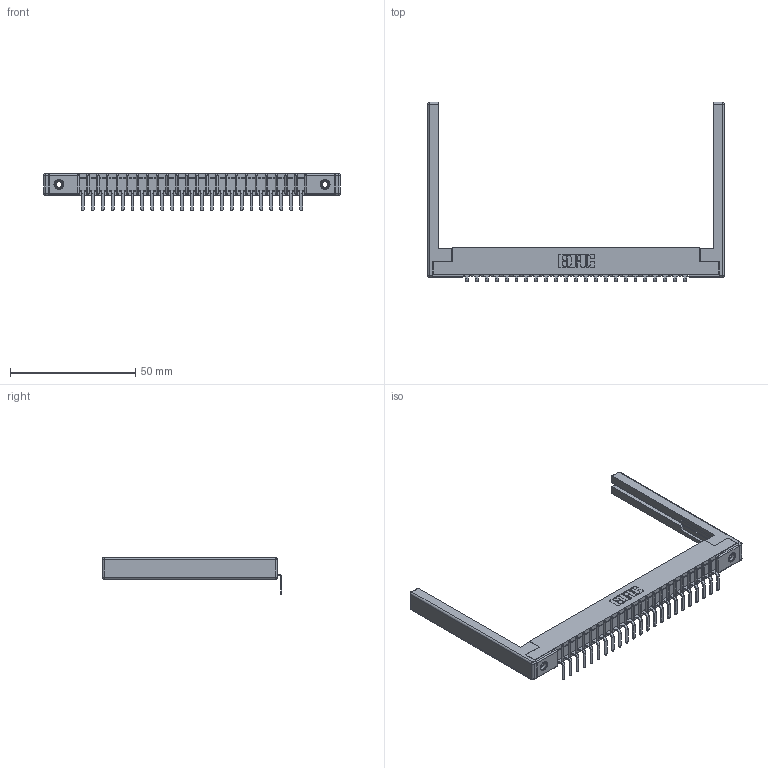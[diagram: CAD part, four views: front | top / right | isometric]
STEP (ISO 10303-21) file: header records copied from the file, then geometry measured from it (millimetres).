
FILE_DESCRIPTION (( 'STEP AP203' ), '1' );
FILE_NAME ('357-023-559-168.STEP', '2022-07-12T22:10:38', ( '' ), ( '' ), 'SwSTEP 2.0', 'SolidWorks 2020', '' );
FILE_SCHEMA (( 'CONFIG_CONTROL_DESIGN' ));
Length unit declared in the file: inch
Products named in the file (5): 307-290-001_558 559 - 1 (Single); 307 Part_.156 Dia Mounting Holes; 345-250-001_345-250-001-102; 357-023-559-168; 307-220-068
Assembly tree (28 placements, depth 2):
  357-023-559-168
    307 Part_.156 Dia Mounting Holes
    307-290-001_558 559 - 1 (Single)  x23
    307-220-068  x2
    345-250-001_345-250-001-102  x2
Bounding box: 118.57 x 71.67 x 14.81 mm (x, y, z)
Volume: 12067.5 mm3; surface area: 15846.9 mm2
Topology: 28 solids, 28 shells, 1676 faces, 4715 edges, 3026 vertices
Faces by surface type: plane 1055, cylinder 549, sphere 56, cone 12, torus 4
Entity records: 24923 total; most frequent: CARTESIAN_POINT 4157, ORIENTED_EDGE 4132, DIRECTION 4072, EDGE_CURVE 2066, VECTOR 1574, LINE 1574, VERTEX_POINT 1334, AXIS2_PLACEMENT_3D 1249
